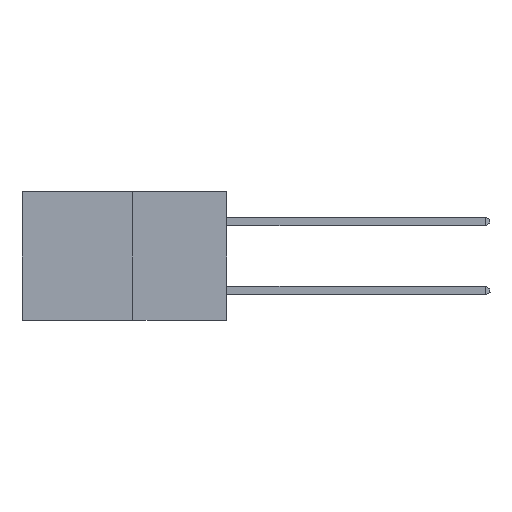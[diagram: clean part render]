
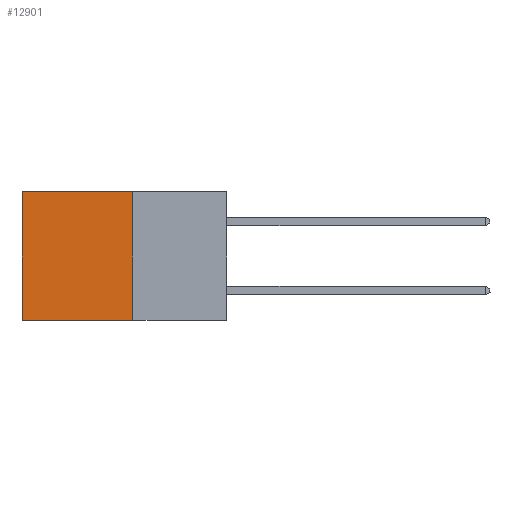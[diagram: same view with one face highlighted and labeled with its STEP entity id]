
A CAD part, left-side view. The second image highlights one B-rep face of the part: STEP entity #12901.
In plain terms, the highlighted planar face has unit normal (-1, 0, 0).
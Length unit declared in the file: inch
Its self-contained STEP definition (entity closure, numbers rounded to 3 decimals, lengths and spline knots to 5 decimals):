
#1507 = CARTESIAN_POINT ( 'NONE',  ( 0.277, 0.27, -0.37 ) ) ;
#1700 = FACE_OUTER_BOUND ( 'NONE', #9154, .T. ) ;
#2434 = PLANE ( 'NONE',  #10819 ) ;
#3867 = ORIENTED_EDGE ( 'NONE', *, *, #23320, .F. ) ;
#4644 = EDGE_CURVE ( 'NONE', #12958, #10560, #21270, .T. ) ;
#5001 = VECTOR ( 'NONE', #5235, 39.37008 ) ;
#5235 = DIRECTION ( 'NONE',  ( 0., 0., -1. ) ) ;
#6232 = DIRECTION ( 'NONE',  ( 1., 0., 0. ) ) ;
#7221 = CARTESIAN_POINT ( 'NONE',  ( 0.277, 0.59, -0.37 ) ) ;
#9154 = EDGE_LOOP ( 'NONE', ( #21324, #3867, #15988, #17423 ) ) ;
#9258 = CARTESIAN_POINT ( 'NONE',  ( 0.277, 0.59, -0.37 ) ) ;
#10021 = LINE ( 'NONE', #12770, #5001 ) ;
#10560 = VERTEX_POINT ( 'NONE', #10861 ) ;
#10819 = AXIS2_PLACEMENT_3D ( 'NONE', #21052, #6232, #19306 ) ;
#10861 = CARTESIAN_POINT ( 'NONE',  ( 0.277, 0.59, 0. ) ) ;
#11843 = VECTOR ( 'NONE', #24063, 39.37008 ) ;
#12027 = CARTESIAN_POINT ( 'NONE',  ( 0.277, 0.27, 0. ) ) ;
#12551 = EDGE_CURVE ( 'NONE', #12958, #16950, #10021, .T. ) ;
#12770 = CARTESIAN_POINT ( 'NONE',  ( 0.277, 0.27, -0.37 ) ) ;
#12862 = DIRECTION ( 'NONE',  ( 0., 1., 0. ) ) ;
#12901 = ADVANCED_FACE ( 'NONE', ( #1700 ), #2434, .F. ) ;
#12958 = VERTEX_POINT ( 'NONE', #12027 ) ;
#15988 = ORIENTED_EDGE ( 'NONE', *, *, #12551, .F. ) ;
#16352 = VECTOR ( 'NONE', #19466, 39.37008 ) ;
#16950 = VERTEX_POINT ( 'NONE', #21990 ) ;
#17423 = ORIENTED_EDGE ( 'NONE', *, *, #4644, .T. ) ;
#19306 = DIRECTION ( 'NONE',  ( 0., 0., -1. ) ) ;
#19466 = DIRECTION ( 'NONE',  ( 0., 1., 0. ) ) ;
#19855 = VECTOR ( 'NONE', #12862, 39.37008 ) ;
#19961 = CARTESIAN_POINT ( 'NONE',  ( 0.277, 0.27, 0. ) ) ;
#20982 = LINE ( 'NONE', #1507, #19855 ) ;
#21052 = CARTESIAN_POINT ( 'NONE',  ( 0.277, 0.27, -0.37 ) ) ;
#21224 = EDGE_CURVE ( 'NONE', #10560, #23899, #21637, .T. ) ;
#21270 = LINE ( 'NONE', #19961, #16352 ) ;
#21324 = ORIENTED_EDGE ( 'NONE', *, *, #21224, .T. ) ;
#21637 = LINE ( 'NONE', #9258, #11843 ) ;
#21990 = CARTESIAN_POINT ( 'NONE',  ( 0.277, 0.27, -0.37 ) ) ;
#23320 = EDGE_CURVE ( 'NONE', #16950, #23899, #20982, .T. ) ;
#23899 = VERTEX_POINT ( 'NONE', #7221 ) ;
#24063 = DIRECTION ( 'NONE',  ( 0., 0., -1. ) ) ;
